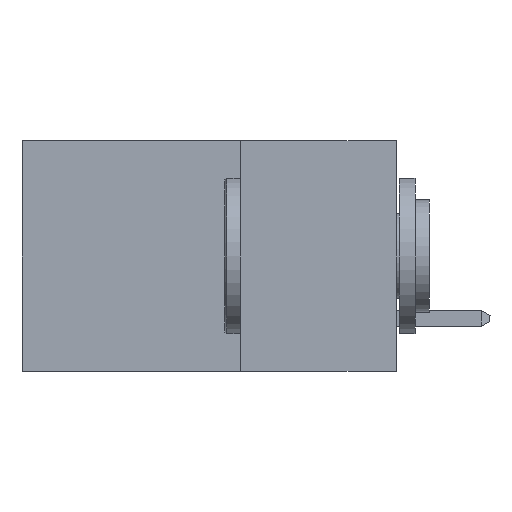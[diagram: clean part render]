
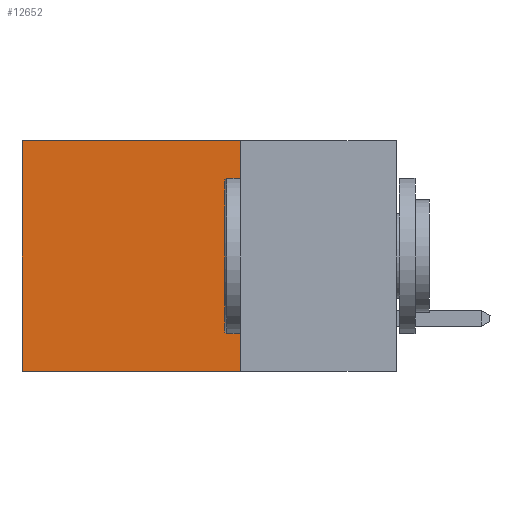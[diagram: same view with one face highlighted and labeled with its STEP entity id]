
A CAD part, left-side view. The second image highlights one B-rep face of the part: STEP entity #12652.
In plain terms, the highlighted planar face has unit normal (-1, 0, 0).
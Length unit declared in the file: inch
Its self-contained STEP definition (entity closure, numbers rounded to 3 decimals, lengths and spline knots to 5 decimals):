
#576 = EDGE_CURVE ( 'NONE', #5082, #4455, #9591, .T. ) ;
#597 = DIRECTION ( 'NONE',  ( 0., 1., 0. ) ) ;
#1143 = FACE_OUTER_BOUND ( 'NONE', #14454, .T. ) ;
#1925 = EDGE_CURVE ( 'NONE', #4455, #17042, #9204, .T. ) ;
#1951 = CARTESIAN_POINT ( 'NONE',  ( 0.2615, 0.25, -0.37 ) ) ;
#1987 = ORIENTED_EDGE ( 'NONE', *, *, #22774, .T. ) ;
#2409 = VECTOR ( 'NONE', #8095, 39.37008 ) ;
#2485 = LINE ( 'NONE', #18296, #7143 ) ;
#2544 = VERTEX_POINT ( 'NONE', #16591 ) ;
#2962 = CARTESIAN_POINT ( 'NONE',  ( 0.2615, 0.6, -0.37 ) ) ;
#2992 = DIRECTION ( 'NONE',  ( 0., 0., -1. ) ) ;
#3741 = DIRECTION ( 'NONE',  ( 0., 1., 0. ) ) ;
#3927 = DIRECTION ( 'NONE',  ( 1., 0., 0. ) ) ;
#4347 = CARTESIAN_POINT ( 'NONE',  ( 0.2615, 0.25, -0.37 ) ) ;
#4455 = VERTEX_POINT ( 'NONE', #13581 ) ;
#5077 = ORIENTED_EDGE ( 'NONE', *, *, #1925, .F. ) ;
#5082 = VERTEX_POINT ( 'NONE', #16523 ) ;
#6089 = CARTESIAN_POINT ( 'NONE',  ( 0.2615, 0.6, -0.37 ) ) ;
#6244 = ORIENTED_EDGE ( 'NONE', *, *, #576, .F. ) ;
#7143 = VECTOR ( 'NONE', #597, 39.37008 ) ;
#7628 = EDGE_CURVE ( 'NONE', #2544, #17042, #17147, .T. ) ;
#8095 = DIRECTION ( 'NONE',  ( 0., 0., -1. ) ) ;
#8589 = VECTOR ( 'NONE', #3741, 39.37008 ) ;
#9204 = LINE ( 'NONE', #4347, #8589 ) ;
#9591 = LINE ( 'NONE', #10564, #2409 ) ;
#10564 = CARTESIAN_POINT ( 'NONE',  ( 0.2615, 0.25, -0.37 ) ) ;
#12652 = ADVANCED_FACE ( 'NONE', ( #1143 ), #13797, .F. ) ;
#13581 = CARTESIAN_POINT ( 'NONE',  ( 0.2615, 0.25, -0.37 ) ) ;
#13797 = PLANE ( 'NONE',  #21925 ) ;
#14454 = EDGE_LOOP ( 'NONE', ( #22168, #5077, #6244, #1987 ) ) ;
#16523 = CARTESIAN_POINT ( 'NONE',  ( 0.2615, 0.25, 0. ) ) ;
#16591 = CARTESIAN_POINT ( 'NONE',  ( 0.2615, 0.6, 0. ) ) ;
#17042 = VERTEX_POINT ( 'NONE', #6089 ) ;
#17147 = LINE ( 'NONE', #2962, #21107 ) ;
#17757 = DIRECTION ( 'NONE',  ( 0., 0., -1. ) ) ;
#18296 = CARTESIAN_POINT ( 'NONE',  ( 0.2615, 0.25, 0. ) ) ;
#21107 = VECTOR ( 'NONE', #2992, 39.37008 ) ;
#21925 = AXIS2_PLACEMENT_3D ( 'NONE', #1951, #3927, #17757 ) ;
#22168 = ORIENTED_EDGE ( 'NONE', *, *, #7628, .T. ) ;
#22774 = EDGE_CURVE ( 'NONE', #5082, #2544, #2485, .T. ) ;
